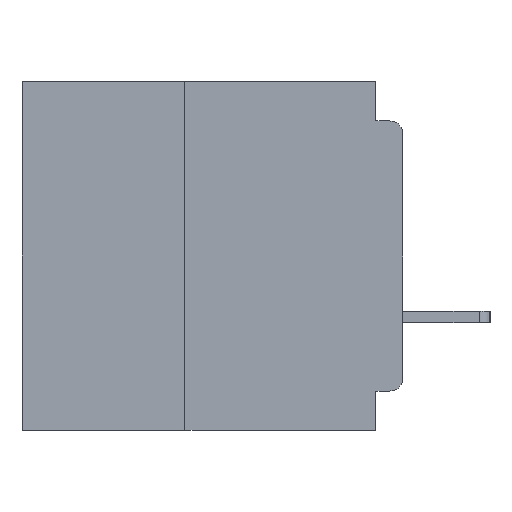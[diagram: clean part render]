
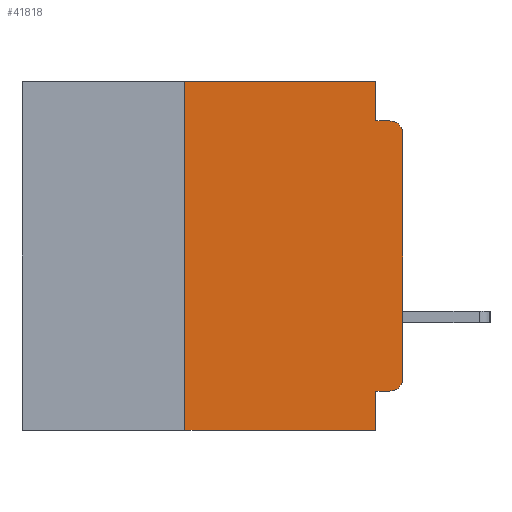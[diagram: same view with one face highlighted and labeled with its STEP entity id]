
A CAD part, left-side view. The second image highlights one B-rep face of the part: STEP entity #41818.
In plain terms, the highlighted planar face has unit normal (-1, 0, 0).
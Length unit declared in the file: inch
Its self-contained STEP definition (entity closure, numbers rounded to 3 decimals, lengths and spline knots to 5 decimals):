
#167 = CARTESIAN_POINT ( 'NONE',  ( 0., 0.437, 0. ) ) ;
#280 = LINE ( 'NONE', #167, #16823 ) ;
#603 = VERTEX_POINT ( 'NONE', #11147 ) ;
#679 = DIRECTION ( 'NONE',  ( 0., 0., 1. ) ) ;
#1255 = VECTOR ( 'NONE', #9841, 39.37008 ) ;
#1888 = LINE ( 'NONE', #32546, #33753 ) ;
#3207 = ORIENTED_EDGE ( 'NONE', *, *, #17371, .F. ) ;
#3495 = EDGE_CURVE ( 'NONE', #40311, #37103, #8851, .T. ) ;
#5299 = VECTOR ( 'NONE', #24356, 39.37008 ) ;
#5321 = EDGE_CURVE ( 'NONE', #7149, #603, #15078, .T. ) ;
#5537 = DIRECTION ( 'NONE',  ( -1., 0., 0. ) ) ;
#6304 = LINE ( 'NONE', #40426, #5299 ) ;
#7086 = CARTESIAN_POINT ( 'NONE',  ( 0., 0.015, -0.045 ) ) ;
#7149 = VERTEX_POINT ( 'NONE', #31869 ) ;
#8271 = VECTOR ( 'NONE', #679, 39.37008 ) ;
#8290 = VERTEX_POINT ( 'NONE', #32189 ) ;
#8851 = CIRCLE ( 'NONE', #13740, 0.015 ) ;
#9276 = LINE ( 'NONE', #39836, #8271 ) ;
#9841 = DIRECTION ( 'NONE',  ( 0., 0., -1. ) ) ;
#10040 = CARTESIAN_POINT ( 'NONE',  ( 0., 0., -0.355 ) ) ;
#10583 = ORIENTED_EDGE ( 'NONE', *, *, #3495, .T. ) ;
#11147 = CARTESIAN_POINT ( 'NONE',  ( 0., 0.031, -0.4 ) ) ;
#11524 = ORIENTED_EDGE ( 'NONE', *, *, #38093, .T. ) ;
#12071 = AXIS2_PLACEMENT_3D ( 'NONE', #25225, #5537, #28508 ) ;
#12391 = ORIENTED_EDGE ( 'NONE', *, *, #34282, .F. ) ;
#12794 = ORIENTED_EDGE ( 'NONE', *, *, #35320, .F. ) ;
#13305 = DIRECTION ( 'NONE',  ( 1., 0., 0. ) ) ;
#13740 = AXIS2_PLACEMENT_3D ( 'NONE', #13790, #36621, #17104 ) ;
#13790 = CARTESIAN_POINT ( 'NONE',  ( 0., 0.015, -0.34 ) ) ;
#15078 = LINE ( 'NONE', #27262, #31479 ) ;
#16002 = ORIENTED_EDGE ( 'NONE', *, *, #34755, .F. ) ;
#16816 = ORIENTED_EDGE ( 'NONE', *, *, #30531, .F. ) ;
#16823 = VECTOR ( 'NONE', #23225, 39.37008 ) ;
#17104 = DIRECTION ( 'NONE',  ( 0., 0., -1. ) ) ;
#17371 = EDGE_CURVE ( 'NONE', #7149, #21109, #9276, .T. ) ;
#20547 = CARTESIAN_POINT ( 'NONE',  ( 0., 0.031, 0. ) ) ;
#20696 = DIRECTION ( 'NONE',  ( 0., -1., 0. ) ) ;
#20790 = CARTESIAN_POINT ( 'NONE',  ( 0., 0.015, -0.355 ) ) ;
#21109 = VERTEX_POINT ( 'NONE', #24804 ) ;
#22941 = VECTOR ( 'NONE', #23256, 39.37008 ) ;
#23225 = DIRECTION ( 'NONE',  ( 0., -1., 0. ) ) ;
#23256 = DIRECTION ( 'NONE',  ( 0., 1., 0. ) ) ;
#23799 = EDGE_CURVE ( 'NONE', #37103, #34916, #40518, .T. ) ;
#24356 = DIRECTION ( 'NONE',  ( 0., -1., 0. ) ) ;
#24804 = CARTESIAN_POINT ( 'NONE',  ( 0., 0.25, 0. ) ) ;
#25225 = CARTESIAN_POINT ( 'NONE',  ( 0., 0.015, -0.06 ) ) ;
#26035 = VERTEX_POINT ( 'NONE', #7086 ) ;
#26468 = LINE ( 'NONE', #42243, #1255 ) ;
#26617 = EDGE_LOOP ( 'NONE', ( #41958, #11524, #16816, #12391, #30230, #3207, #28080, #12794, #16002, #10583 ) ) ;
#27262 = CARTESIAN_POINT ( 'NONE',  ( 0., 0.437, -0.4 ) ) ;
#28080 = ORIENTED_EDGE ( 'NONE', *, *, #5321, .T. ) ;
#28508 = DIRECTION ( 'NONE',  ( 0., 0., -1. ) ) ;
#29384 = DIRECTION ( 'NONE',  ( 0., 0., 1. ) ) ;
#29655 = CARTESIAN_POINT ( 'NONE',  ( 0., 0., -0.34 ) ) ;
#29773 = VERTEX_POINT ( 'NONE', #20547 ) ;
#30230 = ORIENTED_EDGE ( 'NONE', *, *, #37740, .F. ) ;
#30531 = EDGE_CURVE ( 'NONE', #8290, #26035, #6304, .T. ) ;
#30630 = CIRCLE ( 'NONE', #12071, 0.015 ) ;
#31115 = FACE_OUTER_BOUND ( 'NONE', #26617, .T. ) ;
#31479 = VECTOR ( 'NONE', #20696, 39.37008 ) ;
#31869 = CARTESIAN_POINT ( 'NONE',  ( 0., 0.25, -0.4 ) ) ;
#32189 = CARTESIAN_POINT ( 'NONE',  ( 0., 0.031, -0.045 ) ) ;
#32546 = CARTESIAN_POINT ( 'NONE',  ( 0., 0.031, 0. ) ) ;
#32957 = CARTESIAN_POINT ( 'NONE',  ( 0., 0.437, 0. ) ) ;
#33753 = VECTOR ( 'NONE', #38946, 39.37008 ) ;
#34005 = CARTESIAN_POINT ( 'NONE',  ( 0., 0., -0.06 ) ) ;
#34282 = EDGE_CURVE ( 'NONE', #29773, #8290, #1888, .T. ) ;
#34755 = EDGE_CURVE ( 'NONE', #40311, #38148, #40150, .T. ) ;
#34916 = VERTEX_POINT ( 'NONE', #34005 ) ;
#35320 = EDGE_CURVE ( 'NONE', #38148, #603, #26468, .T. ) ;
#36021 = PLANE ( 'NONE',  #38421 ) ;
#36157 = DIRECTION ( 'NONE',  ( 0., 0., -1. ) ) ;
#36621 = DIRECTION ( 'NONE',  ( -1., 0., 0. ) ) ;
#37103 = VERTEX_POINT ( 'NONE', #29655 ) ;
#37740 = EDGE_CURVE ( 'NONE', #21109, #29773, #280, .T. ) ;
#38093 = EDGE_CURVE ( 'NONE', #34916, #26035, #30630, .T. ) ;
#38148 = VERTEX_POINT ( 'NONE', #41550 ) ;
#38421 = AXIS2_PLACEMENT_3D ( 'NONE', #32957, #13305, #36157 ) ;
#38946 = DIRECTION ( 'NONE',  ( 0., 0., -1. ) ) ;
#38947 = CARTESIAN_POINT ( 'NONE',  ( 0., 0., 0. ) ) ;
#39517 = VECTOR ( 'NONE', #29384, 39.37008 ) ;
#39836 = CARTESIAN_POINT ( 'NONE',  ( 0., 0.25, -0.4 ) ) ;
#40150 = LINE ( 'NONE', #10040, #22941 ) ;
#40311 = VERTEX_POINT ( 'NONE', #20790 ) ;
#40426 = CARTESIAN_POINT ( 'NONE',  ( 0., 0., -0.045 ) ) ;
#40518 = LINE ( 'NONE', #38947, #39517 ) ;
#41550 = CARTESIAN_POINT ( 'NONE',  ( 0., 0.031, -0.355 ) ) ;
#41818 = ADVANCED_FACE ( 'NONE', ( #31115 ), #36021, .F. ) ;
#41958 = ORIENTED_EDGE ( 'NONE', *, *, #23799, .T. ) ;
#42243 = CARTESIAN_POINT ( 'NONE',  ( 0., 0.031, -0.4 ) ) ;
